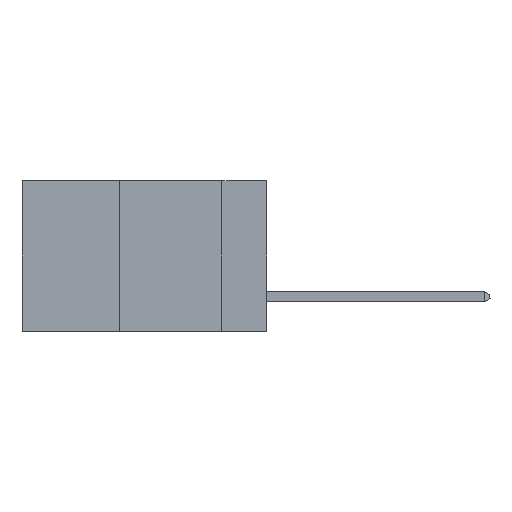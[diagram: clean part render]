
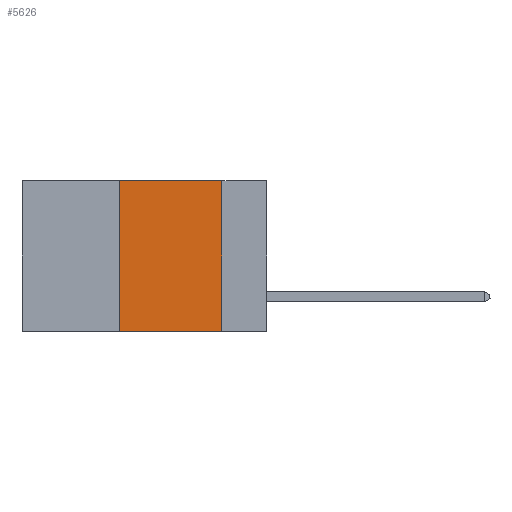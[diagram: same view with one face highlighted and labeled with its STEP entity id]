
A CAD part, left-side view. The second image highlights one B-rep face of the part: STEP entity #5626.
In plain terms, the highlighted planar face has unit normal (-1, 0, 0).
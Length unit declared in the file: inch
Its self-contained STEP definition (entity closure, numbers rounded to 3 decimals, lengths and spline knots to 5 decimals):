
#376 = DIRECTION ( 'NONE',  ( 0., 0., 1. ) ) ;
#444 = CARTESIAN_POINT ( 'NONE',  ( 0., 0.6, -0.37 ) ) ;
#1787 = EDGE_CURVE ( 'NONE', #8594, #2503, #4476, .T. ) ;
#2284 = EDGE_CURVE ( 'NONE', #9128, #8594, #12101, .T. ) ;
#2342 = ORIENTED_EDGE ( 'NONE', *, *, #1787, .F. ) ;
#2503 = VERTEX_POINT ( 'NONE', #7903 ) ;
#2576 = ORIENTED_EDGE ( 'NONE', *, *, #2284, .F. ) ;
#2940 = LINE ( 'NONE', #444, #4872 ) ;
#2979 = CARTESIAN_POINT ( 'NONE',  ( 0., 0.36, -0.37 ) ) ;
#4148 = ORIENTED_EDGE ( 'NONE', *, *, #5868, .F. ) ;
#4251 = EDGE_LOOP ( 'NONE', ( #2342, #2576, #4148, #9789 ) ) ;
#4476 = LINE ( 'NONE', #12740, #9560 ) ;
#4772 = DIRECTION ( 'NONE',  ( 1., 0., 0. ) ) ;
#4872 = VECTOR ( 'NONE', #6605, 39.37008 ) ;
#5262 = CARTESIAN_POINT ( 'NONE',  ( 0., 0.36, 0. ) ) ;
#5347 = VECTOR ( 'NONE', #376, 39.37008 ) ;
#5504 = LINE ( 'NONE', #8577, #5347 ) ;
#5626 = ADVANCED_FACE ( 'NONE', ( #13140 ), #10685, .F. ) ;
#5868 = EDGE_CURVE ( 'NONE', #10216, #9128, #5504, .T. ) ;
#6605 = DIRECTION ( 'NONE',  ( 0., -1., 0. ) ) ;
#7418 = DIRECTION ( 'NONE',  ( 0., -1., 0. ) ) ;
#7449 = VECTOR ( 'NONE', #7418, 39.37008 ) ;
#7562 = CARTESIAN_POINT ( 'NONE',  ( 0., 0.6, 0. ) ) ;
#7903 = CARTESIAN_POINT ( 'NONE',  ( 0., 0.11, -0.37 ) ) ;
#8110 = AXIS2_PLACEMENT_3D ( 'NONE', #10952, #4772, #10869 ) ;
#8577 = CARTESIAN_POINT ( 'NONE',  ( 0., 0.36, 0. ) ) ;
#8594 = VERTEX_POINT ( 'NONE', #11719 ) ;
#9128 = VERTEX_POINT ( 'NONE', #5262 ) ;
#9329 = DIRECTION ( 'NONE',  ( 0., 0., -1. ) ) ;
#9560 = VECTOR ( 'NONE', #9329, 39.37008 ) ;
#9789 = ORIENTED_EDGE ( 'NONE', *, *, #13034, .T. ) ;
#10216 = VERTEX_POINT ( 'NONE', #2979 ) ;
#10685 = PLANE ( 'NONE',  #8110 ) ;
#10869 = DIRECTION ( 'NONE',  ( 0., 0., -1. ) ) ;
#10952 = CARTESIAN_POINT ( 'NONE',  ( 0., 0.6, 0. ) ) ;
#11719 = CARTESIAN_POINT ( 'NONE',  ( 0., 0.11, 0. ) ) ;
#12101 = LINE ( 'NONE', #7562, #7449 ) ;
#12740 = CARTESIAN_POINT ( 'NONE',  ( 0., 0.11, 0. ) ) ;
#13034 = EDGE_CURVE ( 'NONE', #10216, #2503, #2940, .T. ) ;
#13140 = FACE_OUTER_BOUND ( 'NONE', #4251, .T. ) ;
